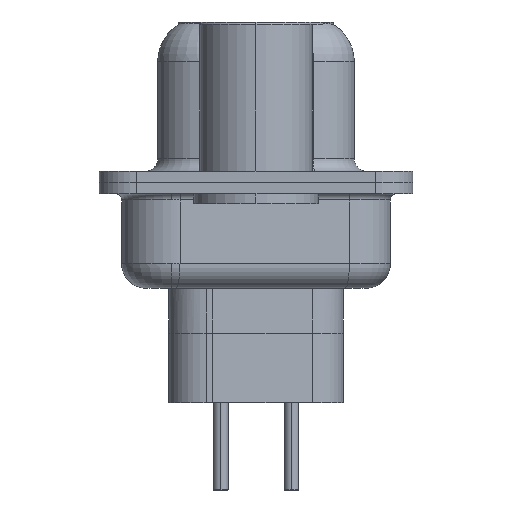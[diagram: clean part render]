
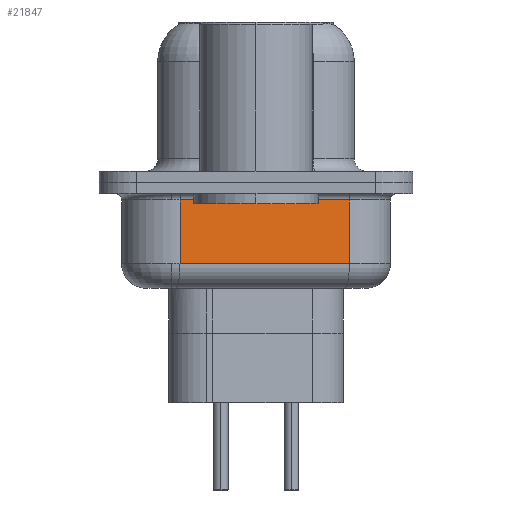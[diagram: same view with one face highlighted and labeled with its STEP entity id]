
A CAD part, left-side view. The second image highlights one B-rep face of the part: STEP entity #21847.
In plain terms, the highlighted planar face has unit normal (-0.985, -0.174, 0).
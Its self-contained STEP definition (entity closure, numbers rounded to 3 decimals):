
#1108 = CARTESIAN_POINT ( 'NONE',  ( 4.074, -3.747, -0.7 ) ) ;
#1774 = VECTOR ( 'NONE', #10382, 1000. ) ;
#4335 = LINE ( 'NONE', #20492, #9841 ) ;
#4479 = VERTEX_POINT ( 'NONE', #7915 ) ;
#4900 = CARTESIAN_POINT ( 'NONE',  ( 2.875, 3.053, -4.25 ) ) ;
#5616 = FACE_OUTER_BOUND ( 'NONE', #20661, .T. ) ;
#5684 = ORIENTED_EDGE ( 'NONE', *, *, #11547, .T. ) ;
#7482 = CARTESIAN_POINT ( 'NONE',  ( 2.875, 3.053, -3.25 ) ) ;
#7638 = DIRECTION ( 'NONE',  ( -0.174, 0.985, 0. ) ) ;
#7862 = ORIENTED_EDGE ( 'NONE', *, *, #21005, .T. ) ;
#7864 = ORIENTED_EDGE ( 'NONE', *, *, #16268, .F. ) ;
#7915 = CARTESIAN_POINT ( 'NONE',  ( 4.074, -3.747, -3.25 ) ) ;
#8483 = DIRECTION ( 'NONE',  ( -0.174, 0.985, 0. ) ) ;
#9741 = EDGE_CURVE ( 'NONE', #4479, #21611, #4335, .T. ) ;
#9841 = VECTOR ( 'NONE', #17068, 1000. ) ;
#9950 = VECTOR ( 'NONE', #8483, 1000. ) ;
#10382 = DIRECTION ( 'NONE',  ( 0., 0., 1. ) ) ;
#11050 = LINE ( 'NONE', #7482, #21676 ) ;
#11431 = CARTESIAN_POINT ( 'NONE',  ( 2.875, 3.053, -4.25 ) ) ;
#11547 = EDGE_CURVE ( 'NONE', #21611, #19639, #22270, .T. ) ;
#11846 = AXIS2_PLACEMENT_3D ( 'NONE', #11431, #16553, #7638 ) ;
#12944 = CARTESIAN_POINT ( 'NONE',  ( 2.875, 3.053, -3.25 ) ) ;
#15527 = ORIENTED_EDGE ( 'NONE', *, *, #9741, .T. ) ;
#15532 = VERTEX_POINT ( 'NONE', #12944 ) ;
#16268 = EDGE_CURVE ( 'NONE', #15532, #19639, #21419, .T. ) ;
#16518 = DIRECTION ( 'NONE',  ( 0.174, -0.985, 0. ) ) ;
#16553 = DIRECTION ( 'NONE',  ( 0.985, 0.174, 0. ) ) ;
#16604 = CARTESIAN_POINT ( 'NONE',  ( 2.875, 3.053, -0.7 ) ) ;
#17068 = DIRECTION ( 'NONE',  ( 0., 0., 1. ) ) ;
#19639 = VERTEX_POINT ( 'NONE', #16604 ) ;
#20104 = PLANE ( 'NONE',  #11846 ) ;
#20492 = CARTESIAN_POINT ( 'NONE',  ( 4.074, -3.747, -4.25 ) ) ;
#20591 = CARTESIAN_POINT ( 'NONE',  ( 2.875, 3.053, -0.7 ) ) ;
#20661 = EDGE_LOOP ( 'NONE', ( #7864, #7862, #15527, #5684 ) ) ;
#21005 = EDGE_CURVE ( 'NONE', #15532, #4479, #11050, .T. ) ;
#21419 = LINE ( 'NONE', #4900, #1774 ) ;
#21611 = VERTEX_POINT ( 'NONE', #1108 ) ;
#21676 = VECTOR ( 'NONE', #16518, 1000. ) ;
#21847 = ADVANCED_FACE ( 'NONE', ( #5616 ), #20104, .F. ) ;
#22270 = LINE ( 'NONE', #20591, #9950 ) ;
